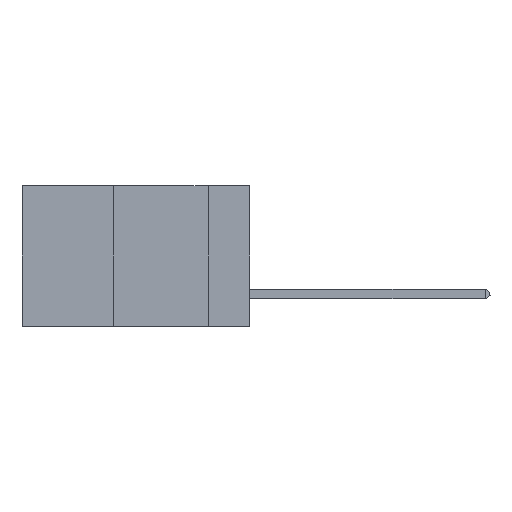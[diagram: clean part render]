
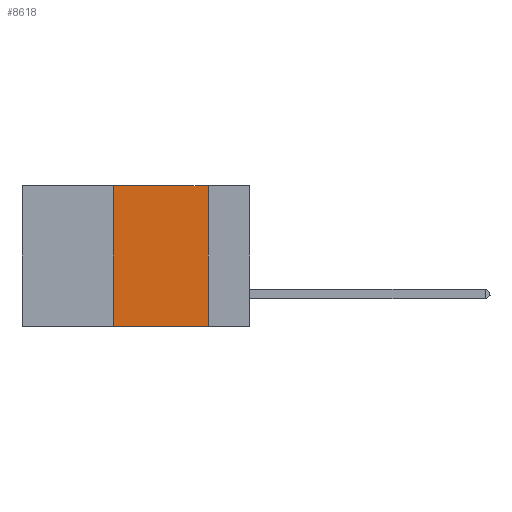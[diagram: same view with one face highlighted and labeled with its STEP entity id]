
A CAD part, left-side view. The second image highlights one B-rep face of the part: STEP entity #8618.
In plain terms, the highlighted planar face has unit normal (-1, 0, 0).
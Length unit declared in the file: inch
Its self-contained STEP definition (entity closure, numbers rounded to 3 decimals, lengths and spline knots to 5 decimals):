
#443 = EDGE_CURVE ( 'NONE', #12913, #16748, #6372, .T. ) ;
#552 = CARTESIAN_POINT ( 'NONE',  ( 0., 0.11, 0. ) ) ;
#1133 = EDGE_CURVE ( 'NONE', #12913, #2077, #3306, .T. ) ;
#1337 = CARTESIAN_POINT ( 'NONE',  ( 0., 0.6, 0. ) ) ;
#2077 = VERTEX_POINT ( 'NONE', #13568 ) ;
#2801 = CARTESIAN_POINT ( 'NONE',  ( 0., 0.6, 0. ) ) ;
#2979 = DIRECTION ( 'NONE',  ( 0., 0., -1. ) ) ;
#3306 = LINE ( 'NONE', #3904, #12539 ) ;
#3528 = CARTESIAN_POINT ( 'NONE',  ( 0., 0.36, 0. ) ) ;
#3904 = CARTESIAN_POINT ( 'NONE',  ( 0., 0.6, -0.37 ) ) ;
#4268 = CARTESIAN_POINT ( 'NONE',  ( 0., 0.11, 0. ) ) ;
#6372 = LINE ( 'NONE', #20885, #11262 ) ;
#6386 = EDGE_CURVE ( 'NONE', #19124, #2077, #8587, .T. ) ;
#6472 = FACE_OUTER_BOUND ( 'NONE', #9489, .T. ) ;
#7510 = ORIENTED_EDGE ( 'NONE', *, *, #443, .F. ) ;
#7816 = VECTOR ( 'NONE', #17374, 39.37008 ) ;
#7987 = DIRECTION ( 'NONE',  ( 0., -1., 0. ) ) ;
#8587 = LINE ( 'NONE', #4268, #7816 ) ;
#8618 = ADVANCED_FACE ( 'NONE', ( #6472 ), #9473, .F. ) ;
#8628 = LINE ( 'NONE', #2801, #17408 ) ;
#9473 = PLANE ( 'NONE',  #14458 ) ;
#9489 = EDGE_LOOP ( 'NONE', ( #16592, #12420, #7510, #18131 ) ) ;
#9696 = DIRECTION ( 'NONE',  ( 0., 0., 1. ) ) ;
#11155 = DIRECTION ( 'NONE',  ( 1., 0., 0. ) ) ;
#11262 = VECTOR ( 'NONE', #9696, 39.37008 ) ;
#12420 = ORIENTED_EDGE ( 'NONE', *, *, #12475, .F. ) ;
#12475 = EDGE_CURVE ( 'NONE', #16748, #19124, #8628, .T. ) ;
#12539 = VECTOR ( 'NONE', #18303, 39.37008 ) ;
#12913 = VERTEX_POINT ( 'NONE', #14022 ) ;
#13568 = CARTESIAN_POINT ( 'NONE',  ( 0., 0.11, -0.37 ) ) ;
#14022 = CARTESIAN_POINT ( 'NONE',  ( 0., 0.36, -0.37 ) ) ;
#14458 = AXIS2_PLACEMENT_3D ( 'NONE', #1337, #11155, #2979 ) ;
#16592 = ORIENTED_EDGE ( 'NONE', *, *, #6386, .F. ) ;
#16748 = VERTEX_POINT ( 'NONE', #3528 ) ;
#17374 = DIRECTION ( 'NONE',  ( 0., 0., -1. ) ) ;
#17408 = VECTOR ( 'NONE', #7987, 39.37008 ) ;
#18131 = ORIENTED_EDGE ( 'NONE', *, *, #1133, .T. ) ;
#18303 = DIRECTION ( 'NONE',  ( 0., -1., 0. ) ) ;
#19124 = VERTEX_POINT ( 'NONE', #552 ) ;
#20885 = CARTESIAN_POINT ( 'NONE',  ( 0., 0.36, 0. ) ) ;
